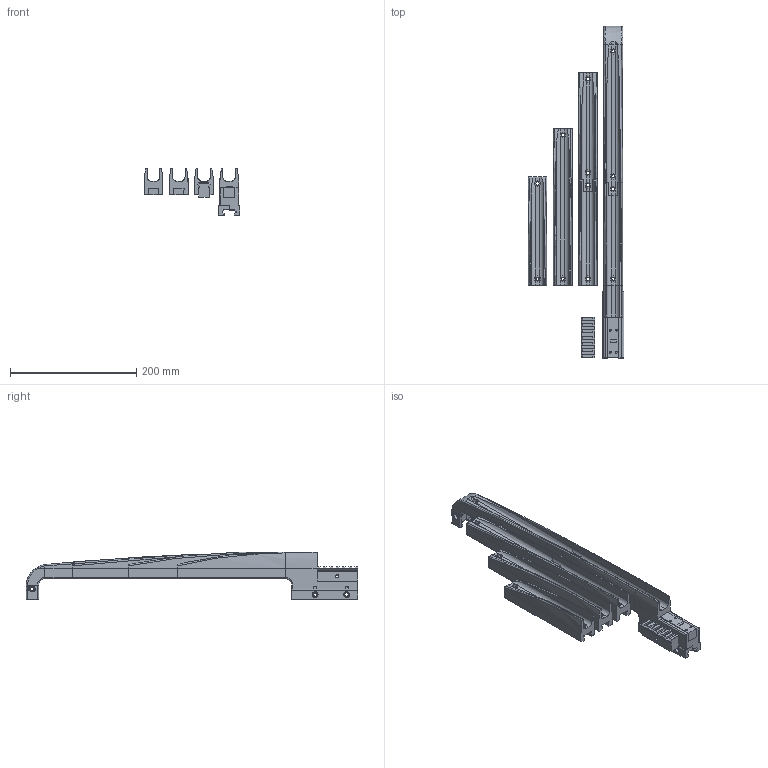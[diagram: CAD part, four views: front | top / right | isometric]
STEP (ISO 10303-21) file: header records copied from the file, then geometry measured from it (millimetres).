
FILE_DESCRIPTION(/* description */ (''),/* implementation_level */ '2;1');
FILE_NAME(/* name */ 'SDI Carry Handle.step',/* time_stamp */ '2022-06-26T18:17:21-05:00',/* author */ (''),/* organization */ (''),/* preprocessor_version */ 'ST-DEVELOPER v19',/* originating_system */ 'Autodesk Translation Framework v11.7.0.108',/* authorisation */ '');
FILE_SCHEMA (('AUTOMOTIVE_DESIGN { 1 0 10303 214 3 1 1 }'));
Length unit declared in the file: millimetre
Products named in the file (1): SDI Carry Handle
Bounding box: 152 x 526 x 76.04 mm (x, y, z)
Volume: 1058788.6 mm3; surface area: 248441.3 mm2
Topology: 12 solids, 12 shells, 707 faces, 1963 edges, 1291 vertices
Faces by surface type: plane 558, cylinder 90, bspline 53, torus 4, sphere 2
Full cylindrical faces by diameter (mm): 3 x4, 4.5 x2, 5 x20, 5.5 x6, 7 x1, 9 x3, 10 x6
Entity records: 26360 total; most frequent: CARTESIAN_POINT 8369, ORIENTED_EDGE 3926, DIRECTION 3372, EDGE_CURVE 1963, LINE 1524, VECTOR 1524, VERTEX_POINT 1291, AXIS2_PLACEMENT_3D 924
